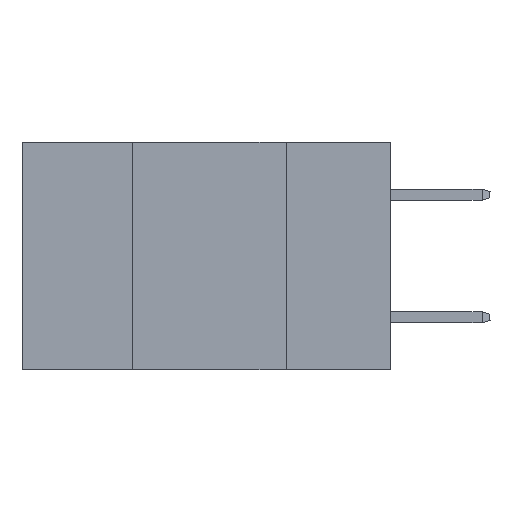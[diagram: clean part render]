
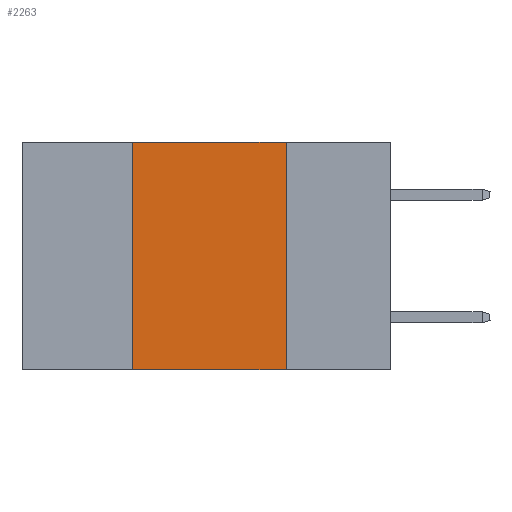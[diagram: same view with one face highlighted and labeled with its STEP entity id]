
A CAD part, left-side view. The second image highlights one B-rep face of the part: STEP entity #2263.
In plain terms, the highlighted planar face has unit normal (-1, 0, 0).
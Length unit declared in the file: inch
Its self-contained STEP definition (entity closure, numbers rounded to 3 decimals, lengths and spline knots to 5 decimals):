
#1125 = PLANE ( 'NONE',  #2494 ) ;
#1362 = ORIENTED_EDGE ( 'NONE', *, *, #7436, .F. ) ;
#1388 = DIRECTION ( 'NONE',  ( 0., 0., -1. ) ) ;
#1782 = CARTESIAN_POINT ( 'NONE',  ( 0., 0.17, 0. ) ) ;
#2095 = LINE ( 'NONE', #6274, #11828 ) ;
#2146 = DIRECTION ( 'NONE',  ( 0., -1., 0. ) ) ;
#2263 = ADVANCED_FACE ( 'NONE', ( #13204 ), #1125, .F. ) ;
#2331 = VERTEX_POINT ( 'NONE', #3039 ) ;
#2494 = AXIS2_PLACEMENT_3D ( 'NONE', #8231, #6911, #1388 ) ;
#2555 = EDGE_CURVE ( 'NONE', #2331, #6309, #14730, .T. ) ;
#3039 = CARTESIAN_POINT ( 'NONE',  ( 0., 0.42, -0.37 ) ) ;
#5362 = VERTEX_POINT ( 'NONE', #5920 ) ;
#5920 = CARTESIAN_POINT ( 'NONE',  ( 0., 0.17, 0. ) ) ;
#6207 = EDGE_CURVE ( 'NONE', #5362, #6309, #11018, .T. ) ;
#6274 = CARTESIAN_POINT ( 'NONE',  ( 0., 0.42, 0. ) ) ;
#6309 = VERTEX_POINT ( 'NONE', #13000 ) ;
#6911 = DIRECTION ( 'NONE',  ( 1., 0., 0. ) ) ;
#7436 = EDGE_CURVE ( 'NONE', #2331, #14171, #2095, .T. ) ;
#7462 = VECTOR ( 'NONE', #2146, 39.37008 ) ;
#7732 = CARTESIAN_POINT ( 'NONE',  ( 0., 0.42, 0. ) ) ;
#8231 = CARTESIAN_POINT ( 'NONE',  ( 0., 0.6, 0. ) ) ;
#8738 = LINE ( 'NONE', #16866, #13561 ) ;
#8875 = ORIENTED_EDGE ( 'NONE', *, *, #6207, .F. ) ;
#8886 = DIRECTION ( 'NONE',  ( 0., 0., -1. ) ) ;
#9696 = VECTOR ( 'NONE', #8886, 39.37008 ) ;
#10568 = CARTESIAN_POINT ( 'NONE',  ( 0., 0.6, -0.37 ) ) ;
#10927 = DIRECTION ( 'NONE',  ( 0., 0., 1. ) ) ;
#11018 = LINE ( 'NONE', #1782, #9696 ) ;
#11157 = ORIENTED_EDGE ( 'NONE', *, *, #2555, .T. ) ;
#11828 = VECTOR ( 'NONE', #10927, 39.37008 ) ;
#12167 = EDGE_LOOP ( 'NONE', ( #8875, #13600, #1362, #11157 ) ) ;
#13000 = CARTESIAN_POINT ( 'NONE',  ( 0., 0.17, -0.37 ) ) ;
#13204 = FACE_OUTER_BOUND ( 'NONE', #12167, .T. ) ;
#13561 = VECTOR ( 'NONE', #14201, 39.37008 ) ;
#13600 = ORIENTED_EDGE ( 'NONE', *, *, #13874, .F. ) ;
#13874 = EDGE_CURVE ( 'NONE', #14171, #5362, #8738, .T. ) ;
#14171 = VERTEX_POINT ( 'NONE', #7732 ) ;
#14201 = DIRECTION ( 'NONE',  ( 0., -1., 0. ) ) ;
#14730 = LINE ( 'NONE', #10568, #7462 ) ;
#16866 = CARTESIAN_POINT ( 'NONE',  ( 0., 0.6, 0. ) ) ;
